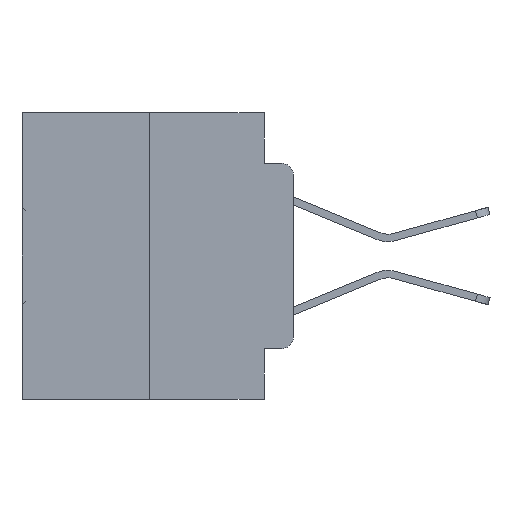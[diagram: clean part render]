
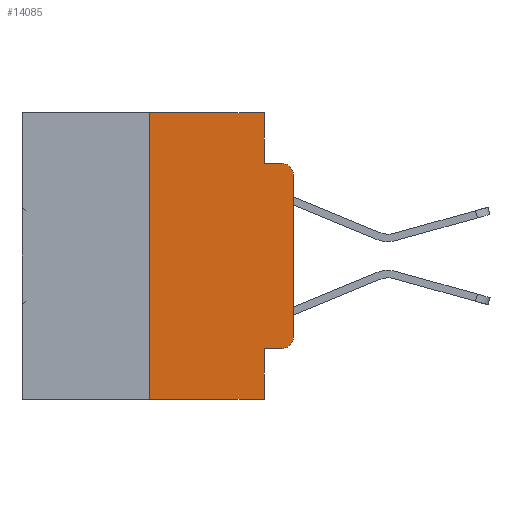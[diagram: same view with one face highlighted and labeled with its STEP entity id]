
A CAD part, left-side view. The second image highlights one B-rep face of the part: STEP entity #14085.
In plain terms, the highlighted planar face has unit normal (-1, 0, 0).
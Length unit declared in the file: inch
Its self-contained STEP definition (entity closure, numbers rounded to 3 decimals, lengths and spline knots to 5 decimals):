
#323 = DIRECTION ( 'NONE',  ( 0., 0., -1. ) ) ;
#784 = ORIENTED_EDGE ( 'NONE', *, *, #16439, .T. ) ;
#1047 = CARTESIAN_POINT ( 'NONE',  ( 0., 0.051, -0.4115 ) ) ;
#1341 = LINE ( 'NONE', #24222, #24710 ) ;
#1344 = AXIS2_PLACEMENT_3D ( 'NONE', #16045, #13764, #323 ) ;
#1437 = CARTESIAN_POINT ( 'NONE',  ( 0., 0.02, -0.3915 ) ) ;
#2376 = VERTEX_POINT ( 'NONE', #7070 ) ;
#2393 = LINE ( 'NONE', #14860, #32380 ) ;
#2592 = VECTOR ( 'NONE', #23527, 39.37008 ) ;
#3332 = DIRECTION ( 'NONE',  ( 0., 0., 1. ) ) ;
#3611 = DIRECTION ( 'NONE',  ( -1., 0., 0. ) ) ;
#4849 = ORIENTED_EDGE ( 'NONE', *, *, #28496, .T. ) ;
#5422 = ORIENTED_EDGE ( 'NONE', *, *, #6690, .F. ) ;
#5956 = DIRECTION ( 'NONE',  ( -1., 0., 0. ) ) ;
#6249 = DIRECTION ( 'NONE',  ( 0., -1., 0. ) ) ;
#6690 = EDGE_CURVE ( 'NONE', #13472, #21275, #1341, .T. ) ;
#6728 = CARTESIAN_POINT ( 'NONE',  ( 0., 0., -0.1085 ) ) ;
#7070 = CARTESIAN_POINT ( 'NONE',  ( 0., 0.02, -0.0885 ) ) ;
#7340 = LINE ( 'NONE', #30892, #18474 ) ;
#7899 = LINE ( 'NONE', #20930, #2592 ) ;
#9793 = EDGE_CURVE ( 'NONE', #23890, #17761, #2393, .T. ) ;
#10482 = VERTEX_POINT ( 'NONE', #14833 ) ;
#10987 = PLANE ( 'NONE',  #1344 ) ;
#11637 = LINE ( 'NONE', #16751, #15778 ) ;
#11813 = DIRECTION ( 'NONE',  ( 0., 0., -1. ) ) ;
#12203 = VERTEX_POINT ( 'NONE', #13617 ) ;
#12404 = FACE_OUTER_BOUND ( 'NONE', #21570, .T. ) ;
#13119 = VECTOR ( 'NONE', #3332, 39.37008 ) ;
#13472 = VERTEX_POINT ( 'NONE', #1047 ) ;
#13563 = DIRECTION ( 'NONE',  ( 0., 0., -1. ) ) ;
#13617 = CARTESIAN_POINT ( 'NONE',  ( 0., 0.25, -0.5 ) ) ;
#13650 = EDGE_CURVE ( 'NONE', #12203, #10482, #7899, .T. ) ;
#13764 = DIRECTION ( 'NONE',  ( 1., 0., 0. ) ) ;
#13805 = CARTESIAN_POINT ( 'NONE',  ( 0., 0., 0. ) ) ;
#13856 = VECTOR ( 'NONE', #15823, 39.37008 ) ;
#13933 = DIRECTION ( 'NONE',  ( 0., -1., 0. ) ) ;
#14065 = CARTESIAN_POINT ( 'NONE',  ( 0., 0.051, -0.0885 ) ) ;
#14085 = ADVANCED_FACE ( 'NONE', ( #12404 ), #10987, .F. ) ;
#14194 = ORIENTED_EDGE ( 'NONE', *, *, #13650, .F. ) ;
#14697 = CIRCLE ( 'NONE', #15929, 0.02 ) ;
#14833 = CARTESIAN_POINT ( 'NONE',  ( 0., 0.25, 0. ) ) ;
#14860 = CARTESIAN_POINT ( 'NONE',  ( 0., 0.051, 0. ) ) ;
#14873 = CIRCLE ( 'NONE', #31278, 0.02 ) ;
#15119 = DIRECTION ( 'NONE',  ( 0., -1., 0. ) ) ;
#15778 = VECTOR ( 'NONE', #13933, 39.37008 ) ;
#15823 = DIRECTION ( 'NONE',  ( 0., -1., 0. ) ) ;
#15929 = AXIS2_PLACEMENT_3D ( 'NONE', #31846, #5956, #13563 ) ;
#16045 = CARTESIAN_POINT ( 'NONE',  ( 0., 0.473, 0. ) ) ;
#16139 = ORIENTED_EDGE ( 'NONE', *, *, #16965, .T. ) ;
#16439 = EDGE_CURVE ( 'NONE', #18948, #2376, #14697, .T. ) ;
#16751 = CARTESIAN_POINT ( 'NONE',  ( 0., 0.473, -0.5 ) ) ;
#16965 = EDGE_CURVE ( 'NONE', #13472, #32248, #18349, .T. ) ;
#17663 = CARTESIAN_POINT ( 'NONE',  ( 0., 0.02, -0.4115 ) ) ;
#17761 = VERTEX_POINT ( 'NONE', #14065 ) ;
#18117 = ORIENTED_EDGE ( 'NONE', *, *, #33114, .F. ) ;
#18349 = LINE ( 'NONE', #28945, #13856 ) ;
#18474 = VECTOR ( 'NONE', #15119, 39.37008 ) ;
#18948 = VERTEX_POINT ( 'NONE', #6728 ) ;
#20582 = VERTEX_POINT ( 'NONE', #21346 ) ;
#20930 = CARTESIAN_POINT ( 'NONE',  ( 0., 0.25, 0. ) ) ;
#21275 = VERTEX_POINT ( 'NONE', #24137 ) ;
#21346 = CARTESIAN_POINT ( 'NONE',  ( 0., 0., -0.3915 ) ) ;
#21360 = ORIENTED_EDGE ( 'NONE', *, *, #9793, .F. ) ;
#21570 = EDGE_LOOP ( 'NONE', ( #22954, #784, #18117, #21360, #33785, #14194, #4849, #5422, #16139, #29462 ) ) ;
#22193 = DIRECTION ( 'NONE',  ( 0., 0., -1. ) ) ;
#22549 = CARTESIAN_POINT ( 'NONE',  ( 0., 0.051, 0. ) ) ;
#22954 = ORIENTED_EDGE ( 'NONE', *, *, #31969, .T. ) ;
#23352 = LINE ( 'NONE', #13805, #13119 ) ;
#23527 = DIRECTION ( 'NONE',  ( 0., 0., 1. ) ) ;
#23890 = VERTEX_POINT ( 'NONE', #22549 ) ;
#24137 = CARTESIAN_POINT ( 'NONE',  ( 0., 0.051, -0.5 ) ) ;
#24222 = CARTESIAN_POINT ( 'NONE',  ( 0., 0.051, 0. ) ) ;
#24710 = VECTOR ( 'NONE', #11813, 39.37008 ) ;
#25406 = DIRECTION ( 'NONE',  ( 0., 0., -1. ) ) ;
#27384 = CARTESIAN_POINT ( 'NONE',  ( 0., 0.051, -0.0885 ) ) ;
#27945 = VECTOR ( 'NONE', #6249, 39.37008 ) ;
#28496 = EDGE_CURVE ( 'NONE', #12203, #21275, #11637, .T. ) ;
#28945 = CARTESIAN_POINT ( 'NONE',  ( 0., 0.051, -0.4115 ) ) ;
#29462 = ORIENTED_EDGE ( 'NONE', *, *, #29683, .T. ) ;
#29576 = LINE ( 'NONE', #27384, #27945 ) ;
#29683 = EDGE_CURVE ( 'NONE', #32248, #20582, #14873, .T. ) ;
#30892 = CARTESIAN_POINT ( 'NONE',  ( 0., 0.473, 0. ) ) ;
#31040 = EDGE_CURVE ( 'NONE', #10482, #23890, #7340, .T. ) ;
#31278 = AXIS2_PLACEMENT_3D ( 'NONE', #1437, #3611, #22193 ) ;
#31846 = CARTESIAN_POINT ( 'NONE',  ( 0., 0.02, -0.1085 ) ) ;
#31969 = EDGE_CURVE ( 'NONE', #20582, #18948, #23352, .T. ) ;
#32248 = VERTEX_POINT ( 'NONE', #17663 ) ;
#32380 = VECTOR ( 'NONE', #25406, 39.37008 ) ;
#33114 = EDGE_CURVE ( 'NONE', #17761, #2376, #29576, .T. ) ;
#33785 = ORIENTED_EDGE ( 'NONE', *, *, #31040, .F. ) ;
